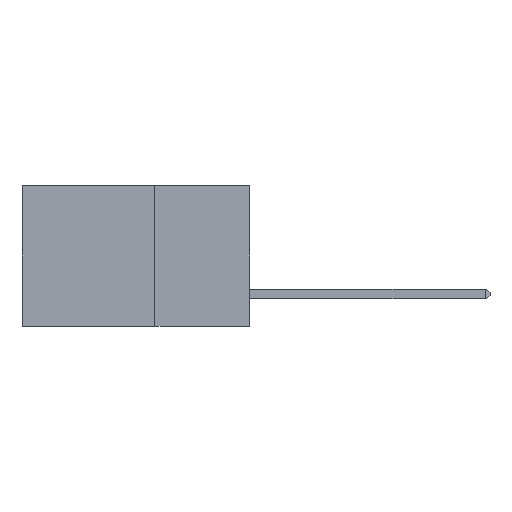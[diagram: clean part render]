
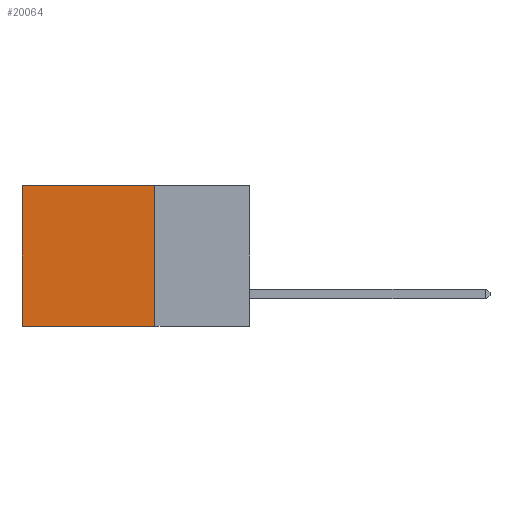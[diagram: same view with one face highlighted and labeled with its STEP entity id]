
A CAD part, left-side view. The second image highlights one B-rep face of the part: STEP entity #20064.
In plain terms, the highlighted planar face has unit normal (-1, 0, 0).
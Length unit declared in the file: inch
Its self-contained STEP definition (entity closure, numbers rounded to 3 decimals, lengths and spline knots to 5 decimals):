
#349 = PLANE ( 'NONE',  #7079 ) ;
#425 = VECTOR ( 'NONE', #12273, 39.37008 ) ;
#431 = DIRECTION ( 'NONE',  ( 1., 0., 0. ) ) ;
#1428 = LINE ( 'NONE', #12497, #10837 ) ;
#1704 = VERTEX_POINT ( 'NONE', #8492 ) ;
#1897 = LINE ( 'NONE', #14522, #11308 ) ;
#1915 = DIRECTION ( 'NONE',  ( 0., 1., 0. ) ) ;
#2047 = CARTESIAN_POINT ( 'NONE',  ( 0.2875, 0.6, 0. ) ) ;
#3025 = ORIENTED_EDGE ( 'NONE', *, *, #16740, .F. ) ;
#3933 = DIRECTION ( 'NONE',  ( 0., 0., -1. ) ) ;
#4431 = ORIENTED_EDGE ( 'NONE', *, *, #5930, .T. ) ;
#5040 = VERTEX_POINT ( 'NONE', #15227 ) ;
#5748 = CARTESIAN_POINT ( 'NONE',  ( 0.2875, 0.25, 0. ) ) ;
#5930 = EDGE_CURVE ( 'NONE', #1704, #5040, #7504, .T. ) ;
#7079 = AXIS2_PLACEMENT_3D ( 'NONE', #5748, #431, #12808 ) ;
#7504 = LINE ( 'NONE', #2047, #21041 ) ;
#8079 = EDGE_LOOP ( 'NONE', ( #4431, #20951, #3025, #18885 ) ) ;
#8269 = CARTESIAN_POINT ( 'NONE',  ( 0.2875, 0.25, 0. ) ) ;
#8492 = CARTESIAN_POINT ( 'NONE',  ( 0.2875, 0.6, 0. ) ) ;
#10494 = CARTESIAN_POINT ( 'NONE',  ( 0.2875, 0.25, 0. ) ) ;
#10837 = VECTOR ( 'NONE', #1915, 39.37008 ) ;
#11308 = VECTOR ( 'NONE', #3933, 39.37008 ) ;
#12273 = DIRECTION ( 'NONE',  ( 0., 1., 0. ) ) ;
#12497 = CARTESIAN_POINT ( 'NONE',  ( 0.2875, 0.25, -0.37 ) ) ;
#12701 = DIRECTION ( 'NONE',  ( 0., 0., -1. ) ) ;
#12808 = DIRECTION ( 'NONE',  ( 0., 0., -1. ) ) ;
#13886 = VERTEX_POINT ( 'NONE', #18265 ) ;
#14522 = CARTESIAN_POINT ( 'NONE',  ( 0.2875, 0.25, 0. ) ) ;
#14782 = VERTEX_POINT ( 'NONE', #8269 ) ;
#15063 = EDGE_CURVE ( 'NONE', #13886, #5040, #1428, .T. ) ;
#15227 = CARTESIAN_POINT ( 'NONE',  ( 0.2875, 0.6, -0.37 ) ) ;
#15987 = FACE_OUTER_BOUND ( 'NONE', #8079, .T. ) ;
#16740 = EDGE_CURVE ( 'NONE', #14782, #13886, #1897, .T. ) ;
#18265 = CARTESIAN_POINT ( 'NONE',  ( 0.2875, 0.25, -0.37 ) ) ;
#18885 = ORIENTED_EDGE ( 'NONE', *, *, #21187, .T. ) ;
#19271 = LINE ( 'NONE', #10494, #425 ) ;
#20064 = ADVANCED_FACE ( 'NONE', ( #15987 ), #349, .F. ) ;
#20951 = ORIENTED_EDGE ( 'NONE', *, *, #15063, .F. ) ;
#21041 = VECTOR ( 'NONE', #12701, 39.37008 ) ;
#21187 = EDGE_CURVE ( 'NONE', #14782, #1704, #19271, .T. ) ;
